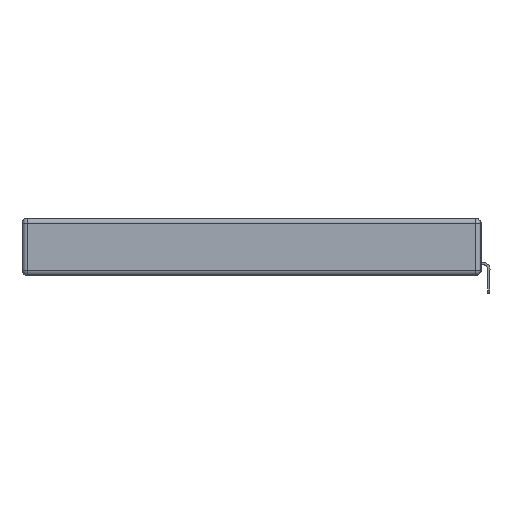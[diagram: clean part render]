
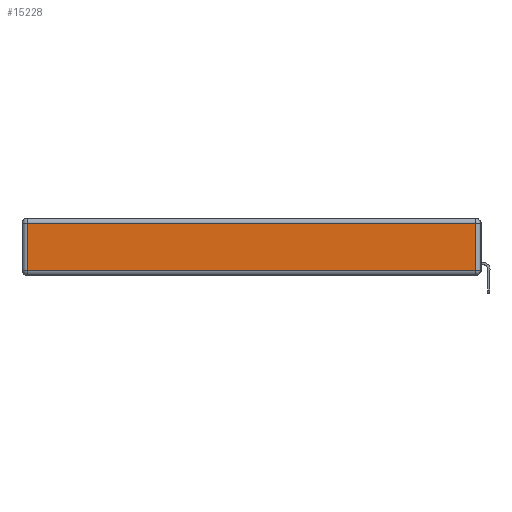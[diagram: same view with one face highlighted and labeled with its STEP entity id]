
A CAD part, left-side view. The second image highlights one B-rep face of the part: STEP entity #15228.
In plain terms, the highlighted planar face has unit normal (-1, 0, 0).
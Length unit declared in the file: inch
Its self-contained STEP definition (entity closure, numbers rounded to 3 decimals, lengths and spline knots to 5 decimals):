
#334 = CARTESIAN_POINT ( 'NONE',  ( 0., 0.03, -0.03 ) ) ;
#772 = CARTESIAN_POINT ( 'NONE',  ( 0., 2.72, -0.313 ) ) ;
#1029 = AXIS2_PLACEMENT_3D ( 'NONE', #3998, #4306, #17438 ) ;
#2468 = PLANE ( 'NONE',  #1029 ) ;
#2537 = EDGE_LOOP ( 'NONE', ( #11604, #17769, #10271, #20093 ) ) ;
#2864 = VERTEX_POINT ( 'NONE', #334 ) ;
#3211 = EDGE_CURVE ( 'NONE', #9421, #2864, #3977, .T. ) ;
#3471 = VECTOR ( 'NONE', #20886, 39.37008 ) ;
#3719 = DIRECTION ( 'NONE',  ( 0., -1., 0. ) ) ;
#3977 = LINE ( 'NONE', #21575, #18339 ) ;
#3998 = CARTESIAN_POINT ( 'NONE',  ( 0., 0., -0.343 ) ) ;
#4242 = LINE ( 'NONE', #14684, #8325 ) ;
#4306 = DIRECTION ( 'NONE',  ( -1., 0., 0. ) ) ;
#5354 = VERTEX_POINT ( 'NONE', #772 ) ;
#5662 = CARTESIAN_POINT ( 'NONE',  ( 0., 0.03, -0.313 ) ) ;
#6681 = DIRECTION ( 'NONE',  ( 0., 1., 0. ) ) ;
#7832 = EDGE_CURVE ( 'NONE', #14706, #5354, #14860, .T. ) ;
#8325 = VECTOR ( 'NONE', #3719, 39.37008 ) ;
#9421 = VERTEX_POINT ( 'NONE', #5662 ) ;
#10271 = ORIENTED_EDGE ( 'NONE', *, *, #15400, .T. ) ;
#11604 = ORIENTED_EDGE ( 'NONE', *, *, #12294, .T. ) ;
#11884 = CARTESIAN_POINT ( 'NONE',  ( 0., 2.72, -0.03 ) ) ;
#12294 = EDGE_CURVE ( 'NONE', #5354, #9421, #4242, .T. ) ;
#13589 = VECTOR ( 'NONE', #6681, 39.37008 ) ;
#14684 = CARTESIAN_POINT ( 'NONE',  ( 0., 0., -0.313 ) ) ;
#14706 = VERTEX_POINT ( 'NONE', #11884 ) ;
#14860 = LINE ( 'NONE', #18923, #3471 ) ;
#15228 = ADVANCED_FACE ( 'NONE', ( #20664 ), #2468, .T. ) ;
#15400 = EDGE_CURVE ( 'NONE', #2864, #14706, #17754, .T. ) ;
#15790 = CARTESIAN_POINT ( 'NONE',  ( 0., 2.75, -0.03 ) ) ;
#17438 = DIRECTION ( 'NONE',  ( 0., 0., 1. ) ) ;
#17754 = LINE ( 'NONE', #15790, #13589 ) ;
#17769 = ORIENTED_EDGE ( 'NONE', *, *, #3211, .T. ) ;
#18339 = VECTOR ( 'NONE', #23263, 39.37008 ) ;
#18923 = CARTESIAN_POINT ( 'NONE',  ( 0., 2.72, -0.343 ) ) ;
#20093 = ORIENTED_EDGE ( 'NONE', *, *, #7832, .T. ) ;
#20664 = FACE_OUTER_BOUND ( 'NONE', #2537, .T. ) ;
#20886 = DIRECTION ( 'NONE',  ( 0., 0., -1. ) ) ;
#21575 = CARTESIAN_POINT ( 'NONE',  ( 0., 0.03, -0.343 ) ) ;
#23263 = DIRECTION ( 'NONE',  ( 0., 0., 1. ) ) ;
